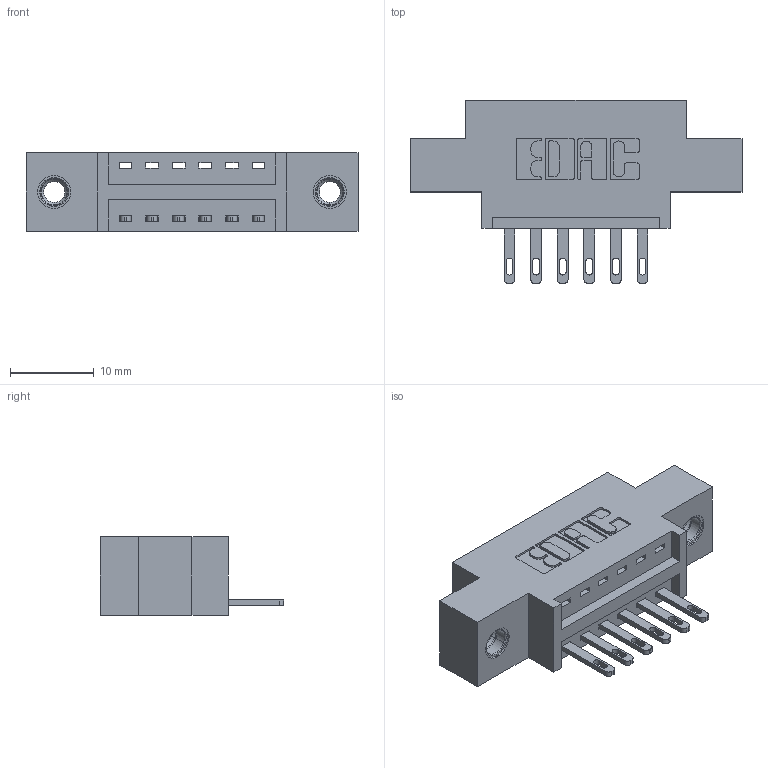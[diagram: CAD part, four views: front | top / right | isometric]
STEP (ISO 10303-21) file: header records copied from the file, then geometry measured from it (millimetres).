
FILE_DESCRIPTION (( 'STEP AP203' ), '1' );
FILE_NAME ('346-006-500-607.STEP', '2018-08-17T02:45:12', ( '' ), ( '' ), 'SwSTEP 2.0', 'SolidWorks 2016', '' );
FILE_SCHEMA (( 'CONFIG_CONTROL_DESIGN' ));
Length unit declared in the file: inch
Products named in the file (4): 345-250-001_345-250-005-103; 346-006-500-607; 346 Part_0.170 Offset - 0.156 Dia-TI; 345-292-001_345-293-100
Assembly tree (9 placements, depth 2):
  346-006-500-607
    346 Part_0.170 Offset - 0.156 Dia-TI
    345-292-001_345-293-100  x6
    345-250-001_345-250-005-103  x2
Bounding box: 39.62 x 21.84 x 9.4 mm (x, y, z)
Volume: 3380.4 mm3; surface area: 4045.6 mm2
Topology: 9 solids, 9 shells, 510 faces, 1485 edges, 982 vertices
Faces by surface type: plane 316, cylinder 178, cone 12, torus 4
Entity records: 9818 total; most frequent: CARTESIAN_POINT 1677, ORIENTED_EDGE 1610, DIRECTION 1551, EDGE_CURVE 805, VECTOR 625, LINE 625, VERTEX_POINT 532, AXIS2_PLACEMENT_3D 463
